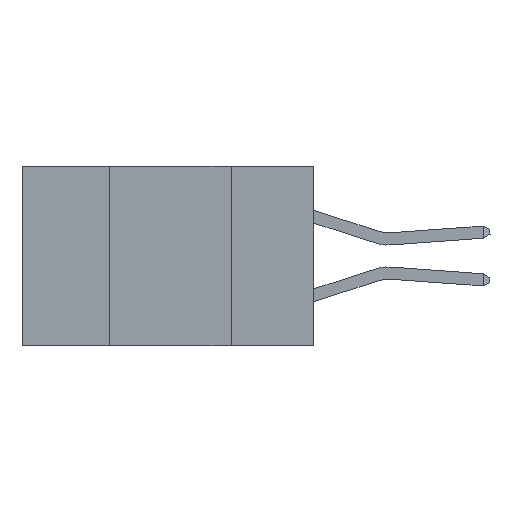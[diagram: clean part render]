
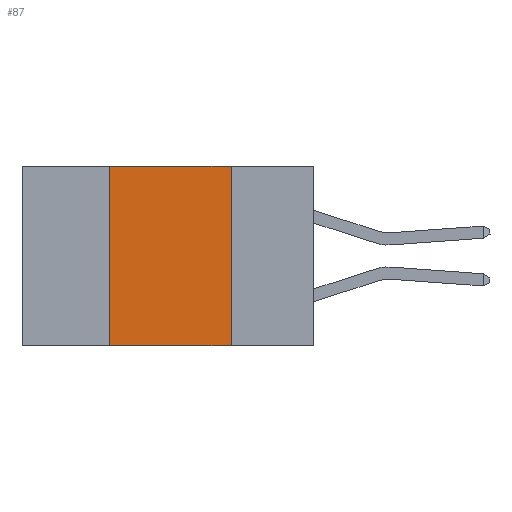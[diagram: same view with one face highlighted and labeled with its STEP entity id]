
A CAD part, left-side view. The second image highlights one B-rep face of the part: STEP entity #87.
In plain terms, the highlighted planar face has unit normal (-1, 0, 0).
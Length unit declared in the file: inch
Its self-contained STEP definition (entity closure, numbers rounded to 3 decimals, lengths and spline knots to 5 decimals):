
#87 = ADVANCED_FACE ( 'NONE', ( #4814 ), #14132, .F. ) ;
#373 = VERTEX_POINT ( 'NONE', #15713 ) ;
#505 = ORIENTED_EDGE ( 'NONE', *, *, #9250, .T. ) ;
#591 = LINE ( 'NONE', #13765, #12453 ) ;
#1906 = DIRECTION ( 'NONE',  ( 0., 0., -1. ) ) ;
#2010 = LINE ( 'NONE', #3182, #9734 ) ;
#2766 = VECTOR ( 'NONE', #8952, 39.37008 ) ;
#3041 = AXIS2_PLACEMENT_3D ( 'NONE', #4874, #17178, #1906 ) ;
#3182 = CARTESIAN_POINT ( 'NONE',  ( 0., 0.6, -0.37 ) ) ;
#4096 = EDGE_CURVE ( 'NONE', #4892, #373, #19221, .T. ) ;
#4814 = FACE_OUTER_BOUND ( 'NONE', #5729, .T. ) ;
#4874 = CARTESIAN_POINT ( 'NONE',  ( 0., 0.6, 0. ) ) ;
#4892 = VERTEX_POINT ( 'NONE', #14727 ) ;
#5580 = VERTEX_POINT ( 'NONE', #17592 ) ;
#5729 = EDGE_LOOP ( 'NONE', ( #10804, #13257, #5748, #505 ) ) ;
#5748 = ORIENTED_EDGE ( 'NONE', *, *, #19920, .F. ) ;
#8952 = DIRECTION ( 'NONE',  ( 0., -1., 0. ) ) ;
#9250 = EDGE_CURVE ( 'NONE', #5580, #11139, #2010, .T. ) ;
#9582 = VECTOR ( 'NONE', #12025, 39.37008 ) ;
#9734 = VECTOR ( 'NONE', #18568, 39.37008 ) ;
#10483 = CARTESIAN_POINT ( 'NONE',  ( 0., 0.17, -0.37 ) ) ;
#10804 = ORIENTED_EDGE ( 'NONE', *, *, #19225, .F. ) ;
#11139 = VERTEX_POINT ( 'NONE', #10483 ) ;
#12007 = LINE ( 'NONE', #19702, #9582 ) ;
#12025 = DIRECTION ( 'NONE',  ( 0., 0., -1. ) ) ;
#12453 = VECTOR ( 'NONE', #16927, 39.37008 ) ;
#13257 = ORIENTED_EDGE ( 'NONE', *, *, #4096, .F. ) ;
#13765 = CARTESIAN_POINT ( 'NONE',  ( 0., 0.42, 0. ) ) ;
#14132 = PLANE ( 'NONE',  #3041 ) ;
#14727 = CARTESIAN_POINT ( 'NONE',  ( 0., 0.42, 0. ) ) ;
#15713 = CARTESIAN_POINT ( 'NONE',  ( 0., 0.17, 0. ) ) ;
#16458 = CARTESIAN_POINT ( 'NONE',  ( 0., 0.6, 0. ) ) ;
#16927 = DIRECTION ( 'NONE',  ( 0., 0., 1. ) ) ;
#17178 = DIRECTION ( 'NONE',  ( 1., 0., 0. ) ) ;
#17592 = CARTESIAN_POINT ( 'NONE',  ( 0., 0.42, -0.37 ) ) ;
#18568 = DIRECTION ( 'NONE',  ( 0., -1., 0. ) ) ;
#19221 = LINE ( 'NONE', #16458, #2766 ) ;
#19225 = EDGE_CURVE ( 'NONE', #373, #11139, #12007, .T. ) ;
#19702 = CARTESIAN_POINT ( 'NONE',  ( 0., 0.17, 0. ) ) ;
#19920 = EDGE_CURVE ( 'NONE', #5580, #4892, #591, .T. ) ;
